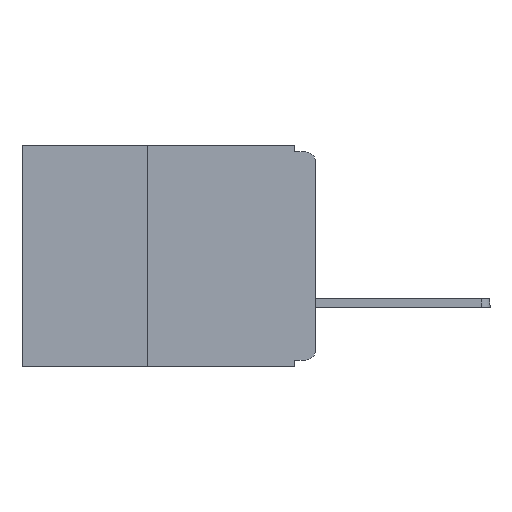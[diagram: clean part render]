
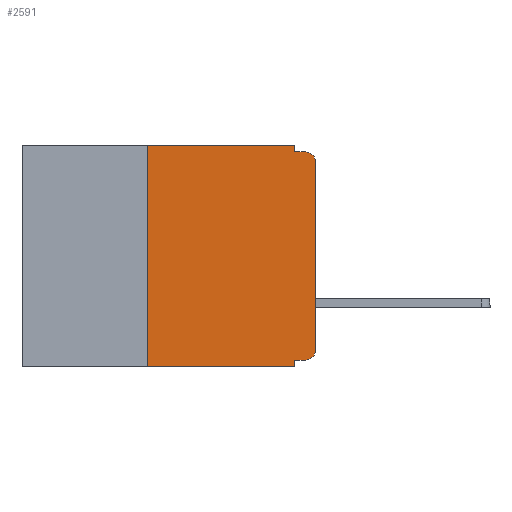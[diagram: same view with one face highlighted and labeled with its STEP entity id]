
A CAD part, left-side view. The second image highlights one B-rep face of the part: STEP entity #2591.
In plain terms, the highlighted planar face has unit normal (-1, 0, 0).
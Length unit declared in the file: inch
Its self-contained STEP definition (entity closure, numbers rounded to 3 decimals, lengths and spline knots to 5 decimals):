
#56 = VERTEX_POINT ( 'NONE', #6467 ) ;
#191 = EDGE_CURVE ( 'NONE', #21182, #20443, #10233, .T. ) ;
#413 = DIRECTION ( 'NONE',  ( 0., -1., 0. ) ) ;
#439 = VECTOR ( 'NONE', #963, 39.37008 ) ;
#511 = VECTOR ( 'NONE', #16488, 39.37008 ) ;
#698 = LINE ( 'NONE', #6204, #9916 ) ;
#933 = VERTEX_POINT ( 'NONE', #22670 ) ;
#963 = DIRECTION ( 'NONE',  ( 0., -1., 0. ) ) ;
#1129 = CARTESIAN_POINT ( 'NONE',  ( 0., 0.031, -0.33 ) ) ;
#2540 = VECTOR ( 'NONE', #18477, 39.37008 ) ;
#2591 = ADVANCED_FACE ( 'NONE', ( #19876 ), #18870, .F. ) ;
#3056 = DIRECTION ( 'NONE',  ( 0., 0., -1. ) ) ;
#3335 = EDGE_CURVE ( 'NONE', #20443, #11636, #14845, .T. ) ;
#3519 = CARTESIAN_POINT ( 'NONE',  ( 0., 0.437, 0. ) ) ;
#3875 = LINE ( 'NONE', #1129, #4426 ) ;
#3980 = VERTEX_POINT ( 'NONE', #17982 ) ;
#4025 = ORIENTED_EDGE ( 'NONE', *, *, #6438, .T. ) ;
#4062 = VERTEX_POINT ( 'NONE', #20188 ) ;
#4355 = DIRECTION ( 'NONE',  ( 0., 1., 0. ) ) ;
#4426 = VECTOR ( 'NONE', #3056, 39.37008 ) ;
#4508 = CARTESIAN_POINT ( 'NONE',  ( 0., 0.25, -0.33 ) ) ;
#4577 = ORIENTED_EDGE ( 'NONE', *, *, #10701, .F. ) ;
#4891 = LINE ( 'NONE', #11348, #14552 ) ;
#5442 = LINE ( 'NONE', #7477, #511 ) ;
#6204 = CARTESIAN_POINT ( 'NONE',  ( 0., 0., -0.32 ) ) ;
#6311 = ORIENTED_EDGE ( 'NONE', *, *, #18124, .T. ) ;
#6363 = DIRECTION ( 'NONE',  ( 0., 0., 1. ) ) ;
#6438 = EDGE_CURVE ( 'NONE', #21644, #3980, #5442, .T. ) ;
#6467 = CARTESIAN_POINT ( 'NONE',  ( 0., 0.015, -0.01 ) ) ;
#7434 = LINE ( 'NONE', #20276, #2540 ) ;
#7477 = CARTESIAN_POINT ( 'NONE',  ( 0., 0., 0. ) ) ;
#7804 = CARTESIAN_POINT ( 'NONE',  ( 0., 0.031, 0. ) ) ;
#8594 = VERTEX_POINT ( 'NONE', #8626 ) ;
#8626 = CARTESIAN_POINT ( 'NONE',  ( 0., 0.25, -0.33 ) ) ;
#9158 = CARTESIAN_POINT ( 'NONE',  ( 0., 0.015, -0.025 ) ) ;
#9455 = ORIENTED_EDGE ( 'NONE', *, *, #3335, .F. ) ;
#9916 = VECTOR ( 'NONE', #4355, 39.37008 ) ;
#10233 = LINE ( 'NONE', #3519, #439 ) ;
#10333 = DIRECTION ( 'NONE',  ( -1., 0., 0. ) ) ;
#10701 = EDGE_CURVE ( 'NONE', #11636, #56, #7434, .T. ) ;
#10985 = DIRECTION ( 'NONE',  ( 0., 0., -1. ) ) ;
#11171 = ORIENTED_EDGE ( 'NONE', *, *, #22535, .F. ) ;
#11348 = CARTESIAN_POINT ( 'NONE',  ( 0., 0.437, -0.33 ) ) ;
#11631 = LINE ( 'NONE', #4508, #16371 ) ;
#11636 = VERTEX_POINT ( 'NONE', #19548 ) ;
#11862 = EDGE_CURVE ( 'NONE', #4062, #933, #698, .T. ) ;
#12067 = CARTESIAN_POINT ( 'NONE',  ( 0., 0.031, 0. ) ) ;
#14060 = DIRECTION ( 'NONE',  ( 0., 0., -1. ) ) ;
#14552 = VECTOR ( 'NONE', #413, 39.37008 ) ;
#14790 = ORIENTED_EDGE ( 'NONE', *, *, #191, .F. ) ;
#14820 = CARTESIAN_POINT ( 'NONE',  ( 0., 0., -0.305 ) ) ;
#14845 = LINE ( 'NONE', #7804, #18984 ) ;
#15893 = ORIENTED_EDGE ( 'NONE', *, *, #11862, .F. ) ;
#16371 = VECTOR ( 'NONE', #6363, 39.37008 ) ;
#16488 = DIRECTION ( 'NONE',  ( 0., 0., 1. ) ) ;
#16717 = CIRCLE ( 'NONE', #16946, 0.015 ) ;
#16946 = AXIS2_PLACEMENT_3D ( 'NONE', #9158, #21612, #10985 ) ;
#17612 = CARTESIAN_POINT ( 'NONE',  ( 0., 0.25, 0. ) ) ;
#17823 = DIRECTION ( 'NONE',  ( 1., 0., 0. ) ) ;
#17982 = CARTESIAN_POINT ( 'NONE',  ( 0., 0., -0.025 ) ) ;
#18124 = EDGE_CURVE ( 'NONE', #8594, #20865, #4891, .T. ) ;
#18477 = DIRECTION ( 'NONE',  ( 0., -1., 0. ) ) ;
#18825 = EDGE_CURVE ( 'NONE', #3980, #56, #16717, .T. ) ;
#18870 = PLANE ( 'NONE',  #20852 ) ;
#18984 = VECTOR ( 'NONE', #14060, 39.37008 ) ;
#19390 = AXIS2_PLACEMENT_3D ( 'NONE', #21001, #10333, #22724 ) ;
#19514 = ORIENTED_EDGE ( 'NONE', *, *, #20370, .F. ) ;
#19548 = CARTESIAN_POINT ( 'NONE',  ( 0., 0.031, -0.01 ) ) ;
#19876 = FACE_OUTER_BOUND ( 'NONE', #23275, .T. ) ;
#20188 = CARTESIAN_POINT ( 'NONE',  ( 0., 0.015, -0.32 ) ) ;
#20276 = CARTESIAN_POINT ( 'NONE',  ( 0., 0., -0.01 ) ) ;
#20370 = EDGE_CURVE ( 'NONE', #8594, #21182, #11631, .T. ) ;
#20443 = VERTEX_POINT ( 'NONE', #12067 ) ;
#20470 = EDGE_CURVE ( 'NONE', #4062, #21644, #22965, .T. ) ;
#20842 = DIRECTION ( 'NONE',  ( 0., 0., -1. ) ) ;
#20852 = AXIS2_PLACEMENT_3D ( 'NONE', #21158, #17823, #20842 ) ;
#20865 = VERTEX_POINT ( 'NONE', #22120 ) ;
#21001 = CARTESIAN_POINT ( 'NONE',  ( 0., 0.015, -0.305 ) ) ;
#21158 = CARTESIAN_POINT ( 'NONE',  ( 0., 0.437, 0. ) ) ;
#21173 = ORIENTED_EDGE ( 'NONE', *, *, #20470, .T. ) ;
#21182 = VERTEX_POINT ( 'NONE', #17612 ) ;
#21612 = DIRECTION ( 'NONE',  ( -1., 0., 0. ) ) ;
#21644 = VERTEX_POINT ( 'NONE', #14820 ) ;
#22120 = CARTESIAN_POINT ( 'NONE',  ( 0., 0.031, -0.33 ) ) ;
#22535 = EDGE_CURVE ( 'NONE', #933, #20865, #3875, .T. ) ;
#22670 = CARTESIAN_POINT ( 'NONE',  ( 0., 0.031, -0.32 ) ) ;
#22724 = DIRECTION ( 'NONE',  ( 0., 0., -1. ) ) ;
#22965 = CIRCLE ( 'NONE', #19390, 0.015 ) ;
#23043 = ORIENTED_EDGE ( 'NONE', *, *, #18825, .T. ) ;
#23275 = EDGE_LOOP ( 'NONE', ( #4025, #23043, #4577, #9455, #14790, #19514, #6311, #11171, #15893, #21173 ) ) ;
